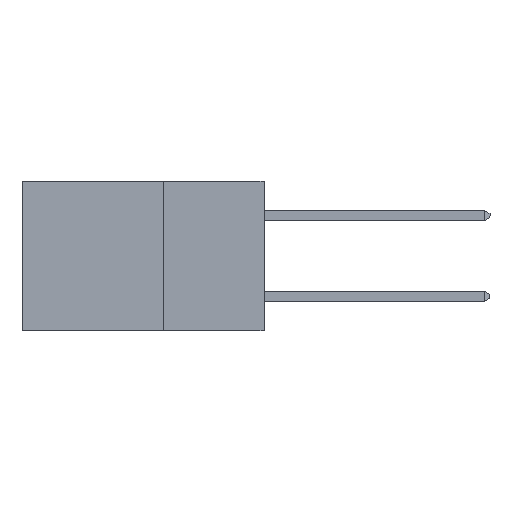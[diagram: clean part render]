
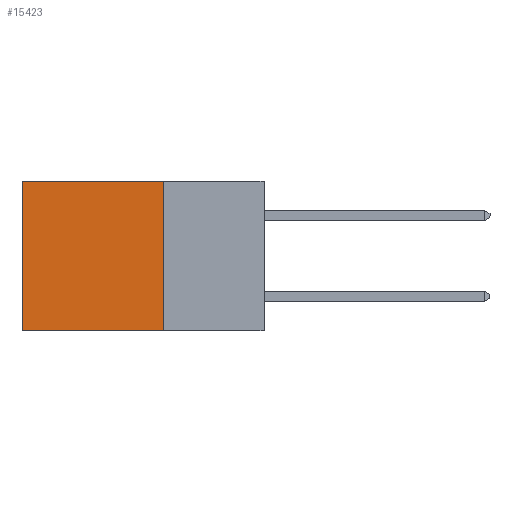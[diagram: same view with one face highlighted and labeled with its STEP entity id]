
A CAD part, left-side view. The second image highlights one B-rep face of the part: STEP entity #15423.
In plain terms, the highlighted planar face has unit normal (-1, 0, 0).
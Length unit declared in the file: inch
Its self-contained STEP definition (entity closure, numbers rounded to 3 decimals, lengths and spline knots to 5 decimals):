
#782 = PLANE ( 'NONE',  #14534 ) ;
#1078 = FACE_OUTER_BOUND ( 'NONE', #4654, .T. ) ;
#1218 = CARTESIAN_POINT ( 'NONE',  ( 0.298, 0.25, -0.37 ) ) ;
#1272 = VECTOR ( 'NONE', #17839, 39.37008 ) ;
#1543 = ORIENTED_EDGE ( 'NONE', *, *, #4577, .F. ) ;
#2363 = VERTEX_POINT ( 'NONE', #21580 ) ;
#2616 = CARTESIAN_POINT ( 'NONE',  ( 0.298, 0.25, 0. ) ) ;
#4377 = LINE ( 'NONE', #5708, #22570 ) ;
#4402 = DIRECTION ( 'NONE',  ( 1., 0., 0. ) ) ;
#4443 = VERTEX_POINT ( 'NONE', #10300 ) ;
#4577 = EDGE_CURVE ( 'NONE', #2363, #10291, #13160, .T. ) ;
#4654 = EDGE_LOOP ( 'NONE', ( #19195, #8198, #1543, #5223 ) ) ;
#5223 = ORIENTED_EDGE ( 'NONE', *, *, #19910, .T. ) ;
#5708 = CARTESIAN_POINT ( 'NONE',  ( 0.298, 0.6, 0. ) ) ;
#6088 = LINE ( 'NONE', #7247, #1272 ) ;
#6383 = DIRECTION ( 'NONE',  ( 0., 0., -1. ) ) ;
#7247 = CARTESIAN_POINT ( 'NONE',  ( 0.298, 0.25, -0.37 ) ) ;
#7598 = DIRECTION ( 'NONE',  ( 0., 1., 0. ) ) ;
#8198 = ORIENTED_EDGE ( 'NONE', *, *, #11114, .F. ) ;
#9565 = VECTOR ( 'NONE', #6383, 39.37008 ) ;
#10170 = CARTESIAN_POINT ( 'NONE',  ( 0.298, 0.25, 0. ) ) ;
#10291 = VERTEX_POINT ( 'NONE', #1218 ) ;
#10300 = CARTESIAN_POINT ( 'NONE',  ( 0.298, 0.6, 0. ) ) ;
#11114 = EDGE_CURVE ( 'NONE', #10291, #14302, #6088, .T. ) ;
#11225 = EDGE_CURVE ( 'NONE', #4443, #14302, #4377, .T. ) ;
#13160 = LINE ( 'NONE', #10170, #9565 ) ;
#14302 = VERTEX_POINT ( 'NONE', #17321 ) ;
#14534 = AXIS2_PLACEMENT_3D ( 'NONE', #2616, #4402, #16801 ) ;
#14584 = DIRECTION ( 'NONE',  ( 0., 0., -1. ) ) ;
#15423 = ADVANCED_FACE ( 'NONE', ( #1078 ), #782, .F. ) ;
#15475 = LINE ( 'NONE', #19935, #20145 ) ;
#16801 = DIRECTION ( 'NONE',  ( 0., 0., -1. ) ) ;
#17321 = CARTESIAN_POINT ( 'NONE',  ( 0.298, 0.6, -0.37 ) ) ;
#17839 = DIRECTION ( 'NONE',  ( 0., 1., 0. ) ) ;
#19195 = ORIENTED_EDGE ( 'NONE', *, *, #11225, .T. ) ;
#19910 = EDGE_CURVE ( 'NONE', #2363, #4443, #15475, .T. ) ;
#19935 = CARTESIAN_POINT ( 'NONE',  ( 0.298, 0.25, 0. ) ) ;
#20145 = VECTOR ( 'NONE', #7598, 39.37008 ) ;
#21580 = CARTESIAN_POINT ( 'NONE',  ( 0.298, 0.25, 0. ) ) ;
#22570 = VECTOR ( 'NONE', #14584, 39.37008 ) ;
